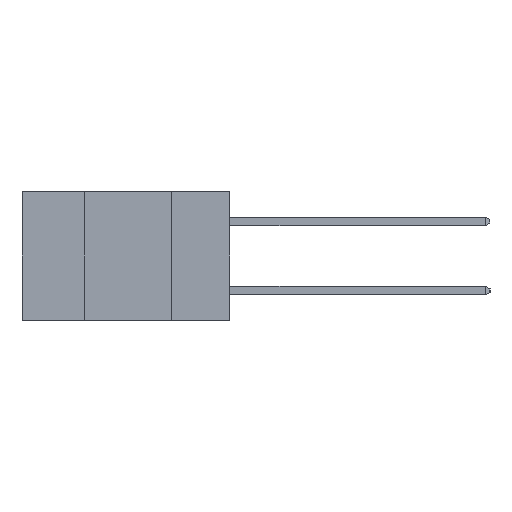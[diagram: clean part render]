
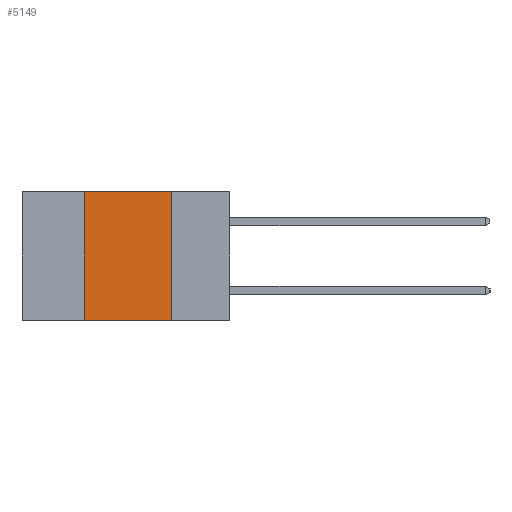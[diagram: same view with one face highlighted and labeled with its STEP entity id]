
A CAD part, left-side view. The second image highlights one B-rep face of the part: STEP entity #5149.
In plain terms, the highlighted planar face has unit normal (-1, 0, 0).
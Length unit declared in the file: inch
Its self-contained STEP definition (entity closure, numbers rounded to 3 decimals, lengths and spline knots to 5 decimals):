
#555 = VERTEX_POINT ( 'NONE', #20807 ) ;
#1332 = DIRECTION ( 'NONE',  ( 0., -1., 0. ) ) ;
#1467 = CARTESIAN_POINT ( 'NONE',  ( 0., 0.6, -0.37 ) ) ;
#2580 = LINE ( 'NONE', #1467, #10672 ) ;
#4183 = VECTOR ( 'NONE', #9507, 39.37008 ) ;
#4841 = DIRECTION ( 'NONE',  ( 0., 0., -1. ) ) ;
#5149 = ADVANCED_FACE ( 'NONE', ( #5800 ), #7947, .F. ) ;
#5515 = VERTEX_POINT ( 'NONE', #19933 ) ;
#5800 = FACE_OUTER_BOUND ( 'NONE', #18914, .T. ) ;
#7472 = DIRECTION ( 'NONE',  ( 0., 0., -1. ) ) ;
#7616 = CARTESIAN_POINT ( 'NONE',  ( 0., 0.6, 0. ) ) ;
#7637 = DIRECTION ( 'NONE',  ( 1., 0., 0. ) ) ;
#7872 = CARTESIAN_POINT ( 'NONE',  ( 0., 0.42, -0.37 ) ) ;
#7947 = PLANE ( 'NONE',  #15626 ) ;
#9048 = CARTESIAN_POINT ( 'NONE',  ( 0., 0.6, 0. ) ) ;
#9507 = DIRECTION ( 'NONE',  ( 0., 0., 1. ) ) ;
#10271 = EDGE_CURVE ( 'NONE', #5515, #13369, #2580, .T. ) ;
#10672 = VECTOR ( 'NONE', #1332, 39.37008 ) ;
#10710 = VECTOR ( 'NONE', #20124, 39.37008 ) ;
#11119 = VECTOR ( 'NONE', #4841, 39.37008 ) ;
#12897 = CARTESIAN_POINT ( 'NONE',  ( 0., 0.17, -0.37 ) ) ;
#13288 = ORIENTED_EDGE ( 'NONE', *, *, #10271, .T. ) ;
#13369 = VERTEX_POINT ( 'NONE', #14670 ) ;
#13426 = ORIENTED_EDGE ( 'NONE', *, *, #19574, .F. ) ;
#13866 = ORIENTED_EDGE ( 'NONE', *, *, #18130, .F. ) ;
#13922 = ORIENTED_EDGE ( 'NONE', *, *, #14991, .F. ) ;
#14670 = CARTESIAN_POINT ( 'NONE',  ( 0., 0.17, -0.37 ) ) ;
#14991 = EDGE_CURVE ( 'NONE', #555, #13369, #15392, .T. ) ;
#15011 = LINE ( 'NONE', #9048, #10710 ) ;
#15279 = VERTEX_POINT ( 'NONE', #18220 ) ;
#15392 = LINE ( 'NONE', #12897, #11119 ) ;
#15626 = AXIS2_PLACEMENT_3D ( 'NONE', #7616, #7637, #7472 ) ;
#16496 = LINE ( 'NONE', #7872, #4183 ) ;
#18130 = EDGE_CURVE ( 'NONE', #15279, #555, #15011, .T. ) ;
#18220 = CARTESIAN_POINT ( 'NONE',  ( 0., 0.42, 0. ) ) ;
#18914 = EDGE_LOOP ( 'NONE', ( #13922, #13866, #13426, #13288 ) ) ;
#19574 = EDGE_CURVE ( 'NONE', #5515, #15279, #16496, .T. ) ;
#19933 = CARTESIAN_POINT ( 'NONE',  ( 0., 0.42, -0.37 ) ) ;
#20124 = DIRECTION ( 'NONE',  ( 0., -1., 0. ) ) ;
#20807 = CARTESIAN_POINT ( 'NONE',  ( 0., 0.17, 0. ) ) ;
